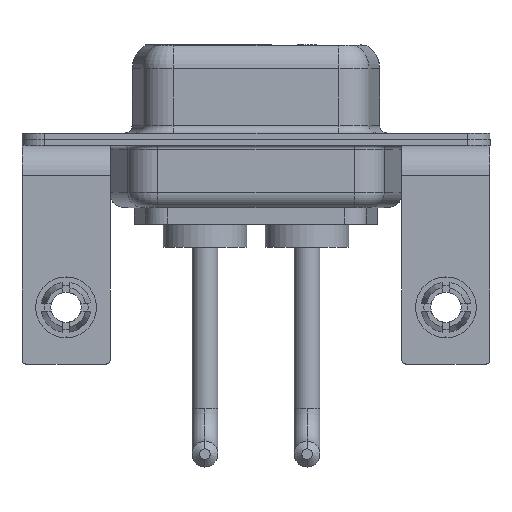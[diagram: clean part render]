
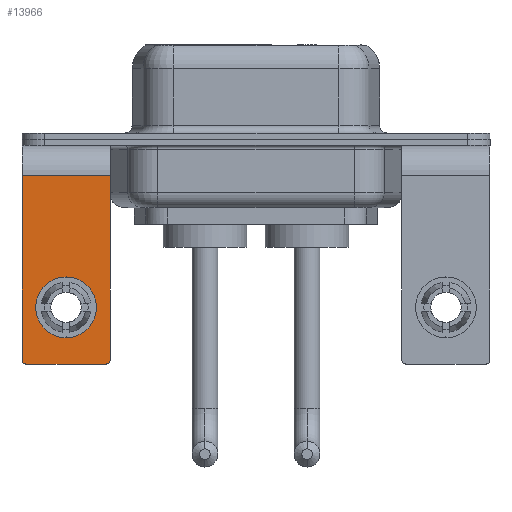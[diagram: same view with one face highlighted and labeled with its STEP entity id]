
A CAD part, front view. The second image highlights one B-rep face of the part: STEP entity #13966.
In plain terms, the highlighted planar face has unit normal (0, -1, 0).
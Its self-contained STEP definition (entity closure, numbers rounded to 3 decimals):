
#121 = FACE_OUTER_BOUND ( 'NONE', #9456, .T. ) ;
#216 = CARTESIAN_POINT ( 'NONE',  ( 0., -6.25, -11.07 ) ) ;
#380 = CARTESIAN_POINT ( 'NONE',  ( 2.9, -6.25, -2.4 ) ) ;
#432 = DIRECTION ( 'NONE',  ( 0., 0., 1. ) ) ;
#474 = DIRECTION ( 'NONE',  ( 0., -1., 0. ) ) ;
#619 = CARTESIAN_POINT ( 'NONE',  ( -2.65, -6.25, -14.8 ) ) ;
#945 = EDGE_LOOP ( 'NONE', ( #2846, #1169 ) ) ;
#952 = EDGE_CURVE ( 'NONE', #10773, #7901, #11549, .T. ) ;
#1169 = ORIENTED_EDGE ( 'NONE', *, *, #2787, .T. ) ;
#1291 = CIRCLE ( 'NONE', #2558, 0.25 ) ;
#1400 = FACE_BOUND ( 'NONE', #945, .T. ) ;
#1679 = CARTESIAN_POINT ( 'NONE',  ( -2.65, -6.25, -14.55 ) ) ;
#1815 = VERTEX_POINT ( 'NONE', #9337 ) ;
#2558 = AXIS2_PLACEMENT_3D ( 'NONE', #5940, #10790, #14271 ) ;
#2747 = DIRECTION ( 'NONE',  ( 0., 1., 0. ) ) ;
#2787 = EDGE_CURVE ( 'NONE', #11035, #11702, #4448, .T. ) ;
#2834 = DIRECTION ( 'NONE',  ( 0., 1., 0. ) ) ;
#2846 = ORIENTED_EDGE ( 'NONE', *, *, #14520, .T. ) ;
#4271 = EDGE_CURVE ( 'NONE', #14772, #10773, #14835, .T. ) ;
#4448 = CIRCLE ( 'NONE', #13317, 2. ) ;
#4930 = DIRECTION ( 'NONE',  ( 0., 1., 0. ) ) ;
#5069 = DIRECTION ( 'NONE',  ( 0., 0., 1. ) ) ;
#5351 = DIRECTION ( 'NONE',  ( 0., 0., 1. ) ) ;
#5814 = VERTEX_POINT ( 'NONE', #619 ) ;
#5940 = CARTESIAN_POINT ( 'NONE',  ( 2.65, -6.25, -14.55 ) ) ;
#6259 = CARTESIAN_POINT ( 'NONE',  ( 2.9, -6.25, -2.4 ) ) ;
#6270 = LINE ( 'NONE', #7618, #8655 ) ;
#6422 = DIRECTION ( 'NONE',  ( -1., 0., 0. ) ) ;
#6991 = CARTESIAN_POINT ( 'NONE',  ( 0., -6.25, -9.07 ) ) ;
#6992 = VERTEX_POINT ( 'NONE', #8693 ) ;
#7105 = ORIENTED_EDGE ( 'NONE', *, *, #12849, .T. ) ;
#7149 = VECTOR ( 'NONE', #8823, 1000. ) ;
#7489 = ORIENTED_EDGE ( 'NONE', *, *, #12532, .F. ) ;
#7618 = CARTESIAN_POINT ( 'NONE',  ( 2.9, -6.25, -14.8 ) ) ;
#7754 = AXIS2_PLACEMENT_3D ( 'NONE', #13715, #2834, #432 ) ;
#7901 = VERTEX_POINT ( 'NONE', #12515 ) ;
#8399 = CARTESIAN_POINT ( 'NONE',  ( 2.9, -6.25, -2.4 ) ) ;
#8655 = VECTOR ( 'NONE', #6422, 1000. ) ;
#8693 = CARTESIAN_POINT ( 'NONE',  ( 2.65, -6.25, -14.8 ) ) ;
#8779 = CIRCLE ( 'NONE', #7754, 2. ) ;
#8823 = DIRECTION ( 'NONE',  ( -1., 0., 0. ) ) ;
#9284 = VECTOR ( 'NONE', #11108, 1000. ) ;
#9337 = CARTESIAN_POINT ( 'NONE',  ( 2.9, -6.25, -14.55 ) ) ;
#9400 = DIRECTION ( 'NONE',  ( 0., 0., -1. ) ) ;
#9456 = EDGE_LOOP ( 'NONE', ( #12238, #11721, #7489, #7105, #11428, #11821 ) ) ;
#9852 = DIRECTION ( 'NONE',  ( 0., 0., 1. ) ) ;
#10201 = CARTESIAN_POINT ( 'NONE',  ( 0., -6.25, -13.07 ) ) ;
#10773 = VERTEX_POINT ( 'NONE', #12315 ) ;
#10790 = DIRECTION ( 'NONE',  ( 0., -1., 0. ) ) ;
#10953 = PLANE ( 'NONE',  #14831 ) ;
#11035 = VERTEX_POINT ( 'NONE', #6991 ) ;
#11108 = DIRECTION ( 'NONE',  ( 0., 0., -1. ) ) ;
#11428 = ORIENTED_EDGE ( 'NONE', *, *, #14530, .F. ) ;
#11549 = LINE ( 'NONE', #15171, #14471 ) ;
#11702 = VERTEX_POINT ( 'NONE', #10201 ) ;
#11721 = ORIENTED_EDGE ( 'NONE', *, *, #15572, .T. ) ;
#11821 = ORIENTED_EDGE ( 'NONE', *, *, #4271, .T. ) ;
#12238 = ORIENTED_EDGE ( 'NONE', *, *, #952, .T. ) ;
#12315 = CARTESIAN_POINT ( 'NONE',  ( -2.9, -6.25, -2.4 ) ) ;
#12366 = CARTESIAN_POINT ( 'NONE',  ( 2.9, -6.25, -2.4 ) ) ;
#12515 = CARTESIAN_POINT ( 'NONE',  ( -2.9, -6.25, -14.55 ) ) ;
#12532 = EDGE_CURVE ( 'NONE', #6992, #5814, #6270, .T. ) ;
#12849 = EDGE_CURVE ( 'NONE', #6992, #1815, #1291, .T. ) ;
#13317 = AXIS2_PLACEMENT_3D ( 'NONE', #216, #4930, #9852 ) ;
#13715 = CARTESIAN_POINT ( 'NONE',  ( 0., -6.25, -11.07 ) ) ;
#13966 = ADVANCED_FACE ( 'NONE', ( #1400, #121 ), #10953, .F. ) ;
#14117 = AXIS2_PLACEMENT_3D ( 'NONE', #1679, #474, #5351 ) ;
#14271 = DIRECTION ( 'NONE',  ( 0., 0., 1. ) ) ;
#14471 = VECTOR ( 'NONE', #9400, 1000. ) ;
#14520 = EDGE_CURVE ( 'NONE', #11702, #11035, #8779, .T. ) ;
#14530 = EDGE_CURVE ( 'NONE', #14772, #1815, #14973, .T. ) ;
#14772 = VERTEX_POINT ( 'NONE', #8399 ) ;
#14831 = AXIS2_PLACEMENT_3D ( 'NONE', #12366, #2747, #5069 ) ;
#14835 = LINE ( 'NONE', #380, #7149 ) ;
#14973 = LINE ( 'NONE', #6259, #9284 ) ;
#15171 = CARTESIAN_POINT ( 'NONE',  ( -2.9, -6.25, -2.4 ) ) ;
#15375 = CIRCLE ( 'NONE', #14117, 0.25 ) ;
#15572 = EDGE_CURVE ( 'NONE', #7901, #5814, #15375, .T. ) ;
